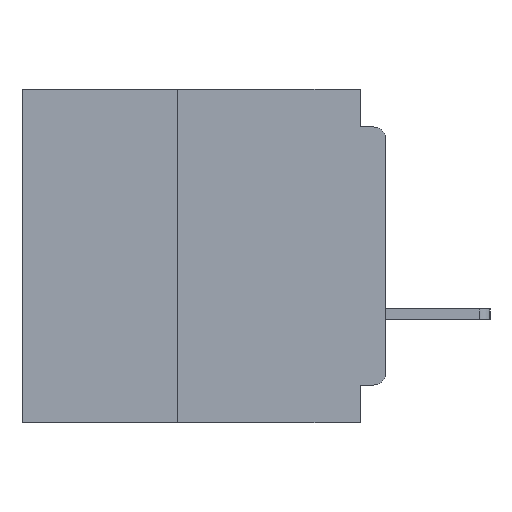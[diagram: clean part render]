
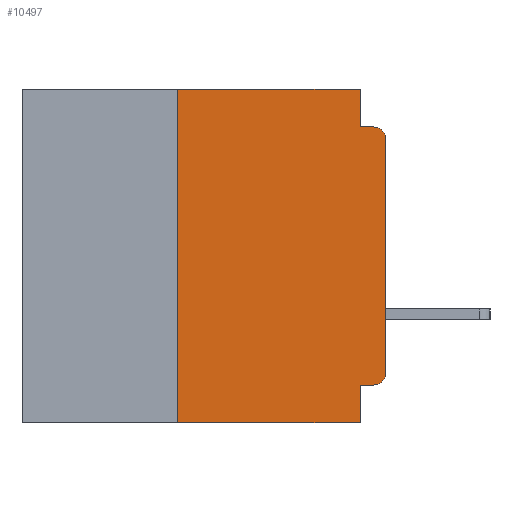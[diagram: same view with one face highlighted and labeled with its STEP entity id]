
A CAD part, left-side view. The second image highlights one B-rep face of the part: STEP entity #10497.
In plain terms, the highlighted planar face has unit normal (-1, 0, 0).
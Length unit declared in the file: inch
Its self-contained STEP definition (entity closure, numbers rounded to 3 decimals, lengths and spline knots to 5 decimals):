
#92 = LINE ( 'NONE', #10112, #28747 ) ;
#794 = ORIENTED_EDGE ( 'NONE', *, *, #3418, .T. ) ;
#855 = DIRECTION ( 'NONE',  ( 0., 0., 1. ) ) ;
#1251 = CARTESIAN_POINT ( 'NONE',  ( 0., 0.031, -0.4 ) ) ;
#2601 = CIRCLE ( 'NONE', #34025, 0.015 ) ;
#3009 = AXIS2_PLACEMENT_3D ( 'NONE', #6450, #25788, #9262 ) ;
#3418 = EDGE_CURVE ( 'NONE', #14882, #28196, #2601, .T. ) ;
#3464 = CARTESIAN_POINT ( 'NONE',  ( 0., 0.25, -0.4 ) ) ;
#3502 = EDGE_LOOP ( 'NONE', ( #9020, #13126, #32771, #14660, #31096, #20216, #25595, #20381, #25016, #794 ) ) ;
#4397 = CARTESIAN_POINT ( 'NONE',  ( 0., 0.437, 0. ) ) ;
#4491 = CARTESIAN_POINT ( 'NONE',  ( 0., 0., -0.355 ) ) ;
#4532 = VERTEX_POINT ( 'NONE', #8993 ) ;
#6450 = CARTESIAN_POINT ( 'NONE',  ( 0., 0.015, -0.06 ) ) ;
#7402 = VERTEX_POINT ( 'NONE', #30490 ) ;
#8046 = CARTESIAN_POINT ( 'NONE',  ( 0., 0., 0. ) ) ;
#8993 = CARTESIAN_POINT ( 'NONE',  ( 0., 0., -0.06 ) ) ;
#9020 = ORIENTED_EDGE ( 'NONE', *, *, #19826, .T. ) ;
#9095 = VERTEX_POINT ( 'NONE', #30777 ) ;
#9262 = DIRECTION ( 'NONE',  ( 0., 0., -1. ) ) ;
#9560 = CARTESIAN_POINT ( 'NONE',  ( 0., 0.015, -0.34 ) ) ;
#9715 = DIRECTION ( 'NONE',  ( 0., 0., -1. ) ) ;
#10043 = DIRECTION ( 'NONE',  ( 1., 0., 0. ) ) ;
#10112 = CARTESIAN_POINT ( 'NONE',  ( 0., 0.031, 0. ) ) ;
#10497 = ADVANCED_FACE ( 'NONE', ( #17686 ), #12736, .F. ) ;
#10823 = CARTESIAN_POINT ( 'NONE',  ( 0., 0., -0.34 ) ) ;
#10992 = DIRECTION ( 'NONE',  ( 0., 0., 1. ) ) ;
#10993 = EDGE_CURVE ( 'NONE', #31887, #25408, #30134, .T. ) ;
#12010 = VECTOR ( 'NONE', #23906, 39.37008 ) ;
#12025 = VERTEX_POINT ( 'NONE', #33786 ) ;
#12371 = DIRECTION ( 'NONE',  ( 0., 0., -1. ) ) ;
#12736 = PLANE ( 'NONE',  #33992 ) ;
#13126 = ORIENTED_EDGE ( 'NONE', *, *, #33166, .T. ) ;
#13476 = VECTOR ( 'NONE', #24602, 39.37008 ) ;
#13671 = EDGE_CURVE ( 'NONE', #7402, #25408, #25812, .T. ) ;
#13709 = LINE ( 'NONE', #8046, #27460 ) ;
#14660 = ORIENTED_EDGE ( 'NONE', *, *, #29832, .F. ) ;
#14882 = VERTEX_POINT ( 'NONE', #20345 ) ;
#15519 = VECTOR ( 'NONE', #20714, 39.37008 ) ;
#15990 = CARTESIAN_POINT ( 'NONE',  ( 0., 0.25, 0. ) ) ;
#17398 = LINE ( 'NONE', #28499, #30248 ) ;
#17686 = FACE_OUTER_BOUND ( 'NONE', #3502, .T. ) ;
#17955 = CARTESIAN_POINT ( 'NONE',  ( 0., 0.437, -0.4 ) ) ;
#18613 = VECTOR ( 'NONE', #23072, 39.37008 ) ;
#19826 = EDGE_CURVE ( 'NONE', #28196, #4532, #13709, .T. ) ;
#20216 = ORIENTED_EDGE ( 'NONE', *, *, #26878, .F. ) ;
#20345 = CARTESIAN_POINT ( 'NONE',  ( 0., 0.015, -0.355 ) ) ;
#20381 = ORIENTED_EDGE ( 'NONE', *, *, #13671, .F. ) ;
#20714 = DIRECTION ( 'NONE',  ( 0., -1., 0. ) ) ;
#21898 = CARTESIAN_POINT ( 'NONE',  ( 0., 0.437, 0. ) ) ;
#22772 = EDGE_CURVE ( 'NONE', #32805, #12025, #28094, .T. ) ;
#23072 = DIRECTION ( 'NONE',  ( 0., -1., 0. ) ) ;
#23906 = DIRECTION ( 'NONE',  ( 0., 1., 0. ) ) ;
#23936 = CARTESIAN_POINT ( 'NONE',  ( 0., 0.015, -0.045 ) ) ;
#24602 = DIRECTION ( 'NONE',  ( 0., -1., 0. ) ) ;
#24960 = VECTOR ( 'NONE', #9715, 39.37008 ) ;
#25016 = ORIENTED_EDGE ( 'NONE', *, *, #29290, .F. ) ;
#25408 = VERTEX_POINT ( 'NONE', #32396 ) ;
#25595 = ORIENTED_EDGE ( 'NONE', *, *, #10993, .T. ) ;
#25665 = CARTESIAN_POINT ( 'NONE',  ( 0., 0., -0.045 ) ) ;
#25785 = LINE ( 'NONE', #4491, #12010 ) ;
#25788 = DIRECTION ( 'NONE',  ( -1., 0., 0. ) ) ;
#25812 = LINE ( 'NONE', #1251, #24960 ) ;
#26878 = EDGE_CURVE ( 'NONE', #31887, #32805, #17398, .T. ) ;
#27460 = VECTOR ( 'NONE', #10992, 39.37008 ) ;
#27566 = LINE ( 'NONE', #25665, #18613 ) ;
#27572 = CIRCLE ( 'NONE', #3009, 0.015 ) ;
#27818 = EDGE_CURVE ( 'NONE', #9095, #35340, #27566, .T. ) ;
#28094 = LINE ( 'NONE', #21898, #13476 ) ;
#28196 = VERTEX_POINT ( 'NONE', #10823 ) ;
#28499 = CARTESIAN_POINT ( 'NONE',  ( 0., 0.25, -0.4 ) ) ;
#28747 = VECTOR ( 'NONE', #29384, 39.37008 ) ;
#28837 = DIRECTION ( 'NONE',  ( -1., 0., 0. ) ) ;
#29290 = EDGE_CURVE ( 'NONE', #14882, #7402, #25785, .T. ) ;
#29316 = DIRECTION ( 'NONE',  ( 0., 0., -1. ) ) ;
#29384 = DIRECTION ( 'NONE',  ( 0., 0., -1. ) ) ;
#29832 = EDGE_CURVE ( 'NONE', #12025, #9095, #92, .T. ) ;
#30134 = LINE ( 'NONE', #17955, #15519 ) ;
#30248 = VECTOR ( 'NONE', #855, 39.37008 ) ;
#30490 = CARTESIAN_POINT ( 'NONE',  ( 0., 0.031, -0.355 ) ) ;
#30777 = CARTESIAN_POINT ( 'NONE',  ( 0., 0.031, -0.045 ) ) ;
#31096 = ORIENTED_EDGE ( 'NONE', *, *, #22772, .F. ) ;
#31887 = VERTEX_POINT ( 'NONE', #3464 ) ;
#32396 = CARTESIAN_POINT ( 'NONE',  ( 0., 0.031, -0.4 ) ) ;
#32771 = ORIENTED_EDGE ( 'NONE', *, *, #27818, .F. ) ;
#32805 = VERTEX_POINT ( 'NONE', #15990 ) ;
#33166 = EDGE_CURVE ( 'NONE', #4532, #35340, #27572, .T. ) ;
#33786 = CARTESIAN_POINT ( 'NONE',  ( 0., 0.031, 0. ) ) ;
#33992 = AXIS2_PLACEMENT_3D ( 'NONE', #4397, #10043, #29316 ) ;
#34025 = AXIS2_PLACEMENT_3D ( 'NONE', #9560, #28837, #12371 ) ;
#35340 = VERTEX_POINT ( 'NONE', #23936 ) ;
